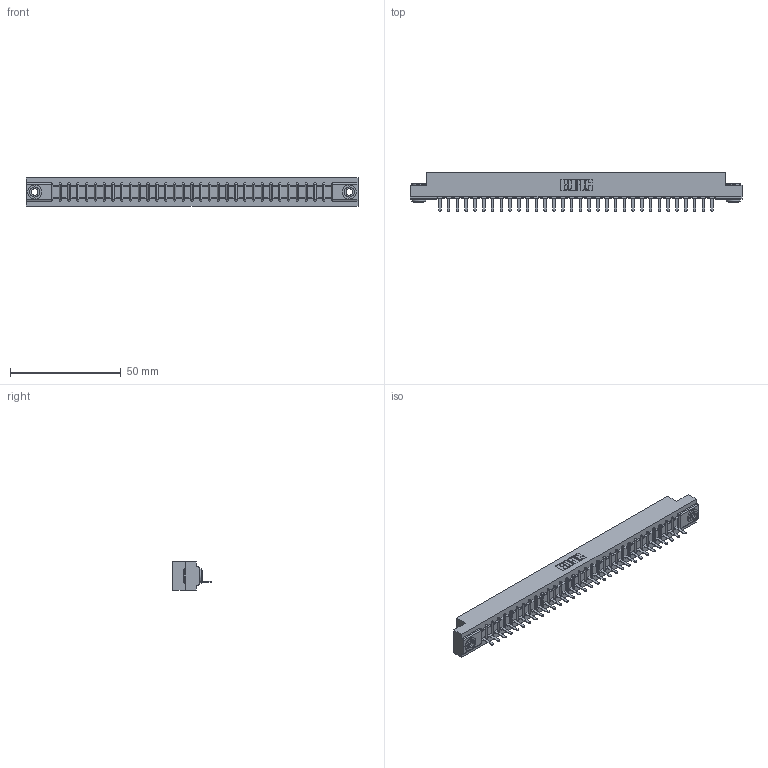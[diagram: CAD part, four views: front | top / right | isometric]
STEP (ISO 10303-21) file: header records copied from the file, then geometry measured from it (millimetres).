
FILE_DESCRIPTION (( 'STEP AP203' ), '1' );
FILE_NAME ('307-032-521-103.STEP', '2019-09-05T05:15:07', ( '' ), ( '' ), 'SwSTEP 2.0', 'SolidWorks 2016', '' );
FILE_SCHEMA (( 'CONFIG_CONTROL_DESIGN' ));
Length unit declared in the file: inch
Products named in the file (4): 307 Part_.156 Dia Mounting Holes; 307-032-521-103; 345-250-002_345-250-002-102; 307-290-002_521
Assembly tree (35 placements, depth 2):
  307-032-521-103
    307 Part_.156 Dia Mounting Holes
    307-290-002_521  x32
    345-250-002_345-250-002-102  x2
Bounding box: 149.81 x 17.42 x 12.7 mm (x, y, z)
Volume: 15960.1 mm3; surface area: 20103.2 mm2
Topology: 35 solids, 35 shells, 2571 faces, 7859 edges, 5146 vertices
Faces by surface type: plane 1534, cylinder 963, sphere 66, cone 8
Entity records: 30449 total; most frequent: CARTESIAN_POINT 5113, ORIENTED_EDGE 5094, DIRECTION 4987, EDGE_CURVE 2547, VECTOR 1939, LINE 1939, VERTEX_POINT 1650, AXIS2_PLACEMENT_3D 1524
